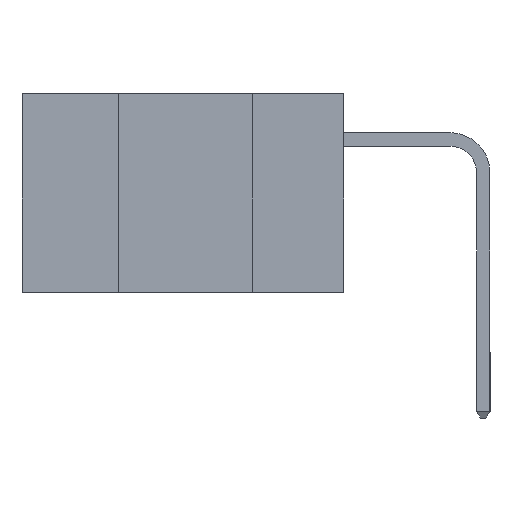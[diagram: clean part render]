
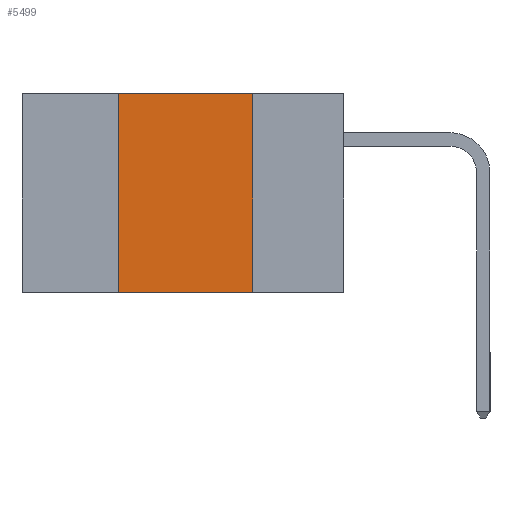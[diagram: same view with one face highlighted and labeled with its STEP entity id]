
A CAD part, left-side view. The second image highlights one B-rep face of the part: STEP entity #5499.
In plain terms, the highlighted planar face has unit normal (-1, 0, 0).
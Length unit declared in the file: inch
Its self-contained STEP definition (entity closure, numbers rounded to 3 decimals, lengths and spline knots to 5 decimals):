
#359 = PLANE ( 'NONE',  #4609 ) ;
#1153 = VERTEX_POINT ( 'NONE', #9393 ) ;
#1816 = CARTESIAN_POINT ( 'NONE',  ( 0., 0.17, 0. ) ) ;
#2097 = LINE ( 'NONE', #1816, #6514 ) ;
#2115 = CARTESIAN_POINT ( 'NONE',  ( 0., 0.42, 0. ) ) ;
#2610 = EDGE_CURVE ( 'NONE', #1153, #19444, #12479, .T. ) ;
#3610 = ORIENTED_EDGE ( 'NONE', *, *, #2610, .F. ) ;
#3616 = DIRECTION ( 'NONE',  ( 0., 0., -1. ) ) ;
#4167 = VECTOR ( 'NONE', #7164, 39.37008 ) ;
#4609 = AXIS2_PLACEMENT_3D ( 'NONE', #16904, #11960, #16834 ) ;
#5251 = DIRECTION ( 'NONE',  ( 0., 0., 1. ) ) ;
#5499 = ADVANCED_FACE ( 'NONE', ( #21248 ), #359, .F. ) ;
#6514 = VECTOR ( 'NONE', #3616, 39.37008 ) ;
#7164 = DIRECTION ( 'NONE',  ( 0., -1., 0. ) ) ;
#7391 = CARTESIAN_POINT ( 'NONE',  ( 0., 0.42, -0.37 ) ) ;
#8902 = ORIENTED_EDGE ( 'NONE', *, *, #20408, .T. ) ;
#8958 = VERTEX_POINT ( 'NONE', #7391 ) ;
#9362 = ORIENTED_EDGE ( 'NONE', *, *, #11727, .F. ) ;
#9393 = CARTESIAN_POINT ( 'NONE',  ( 0., 0.42, 0. ) ) ;
#9652 = EDGE_CURVE ( 'NONE', #8958, #1153, #19391, .T. ) ;
#11303 = VECTOR ( 'NONE', #5251, 39.37008 ) ;
#11548 = VERTEX_POINT ( 'NONE', #11610 ) ;
#11610 = CARTESIAN_POINT ( 'NONE',  ( 0., 0.17, -0.37 ) ) ;
#11691 = VECTOR ( 'NONE', #13987, 39.37008 ) ;
#11727 = EDGE_CURVE ( 'NONE', #19444, #11548, #2097, .T. ) ;
#11960 = DIRECTION ( 'NONE',  ( 1., 0., 0. ) ) ;
#12328 = CARTESIAN_POINT ( 'NONE',  ( 0., 0.6, 0. ) ) ;
#12479 = LINE ( 'NONE', #12328, #11691 ) ;
#13467 = CARTESIAN_POINT ( 'NONE',  ( 0., 0.17, 0. ) ) ;
#13987 = DIRECTION ( 'NONE',  ( 0., -1., 0. ) ) ;
#15665 = CARTESIAN_POINT ( 'NONE',  ( 0., 0.6, -0.37 ) ) ;
#16834 = DIRECTION ( 'NONE',  ( 0., 0., -1. ) ) ;
#16904 = CARTESIAN_POINT ( 'NONE',  ( 0., 0.6, 0. ) ) ;
#19180 = ORIENTED_EDGE ( 'NONE', *, *, #9652, .F. ) ;
#19391 = LINE ( 'NONE', #2115, #11303 ) ;
#19444 = VERTEX_POINT ( 'NONE', #13467 ) ;
#20336 = LINE ( 'NONE', #15665, #4167 ) ;
#20408 = EDGE_CURVE ( 'NONE', #8958, #11548, #20336, .T. ) ;
#20673 = EDGE_LOOP ( 'NONE', ( #9362, #3610, #19180, #8902 ) ) ;
#21248 = FACE_OUTER_BOUND ( 'NONE', #20673, .T. ) ;
